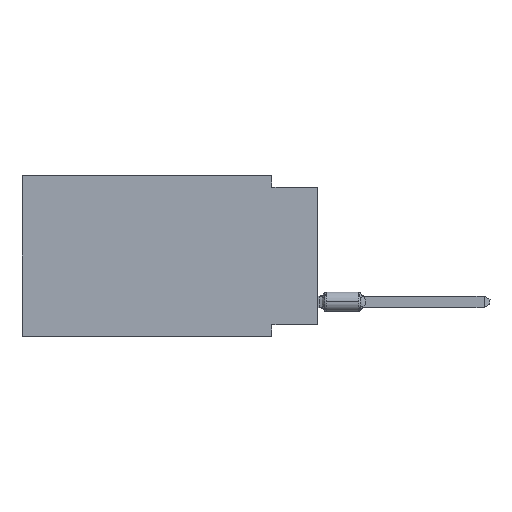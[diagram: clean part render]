
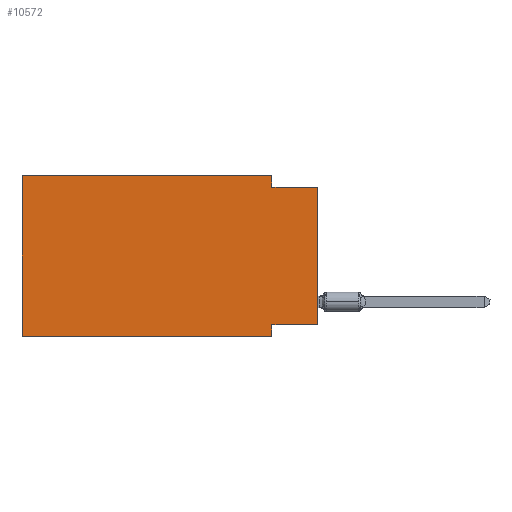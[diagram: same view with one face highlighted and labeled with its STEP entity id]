
A CAD part, left-side view. The second image highlights one B-rep face of the part: STEP entity #10572.
In plain terms, the highlighted planar face has unit normal (-1, 0, 0).
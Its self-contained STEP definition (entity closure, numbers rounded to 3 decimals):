
#329 = ORIENTED_EDGE ( 'NONE', *, *, #6114, .F. ) ;
#691 = DIRECTION ( 'NONE',  ( 1., 0., 0. ) ) ;
#1422 = CARTESIAN_POINT ( 'NONE',  ( 0., 0., -8.255 ) ) ;
#1438 = DIRECTION ( 'NONE',  ( 0., 0., 1. ) ) ;
#2077 = CARTESIAN_POINT ( 'NONE',  ( 0., 2.54, -0.635 ) ) ;
#2376 = EDGE_CURVE ( 'NONE', #9043, #14694, #4723, .T. ) ;
#2494 = VERTEX_POINT ( 'NONE', #3031 ) ;
#2720 = CARTESIAN_POINT ( 'NONE',  ( 0., 2.54, 0. ) ) ;
#2972 = LINE ( 'NONE', #18921, #23344 ) ;
#3031 = CARTESIAN_POINT ( 'NONE',  ( 0., 0., -8.255 ) ) ;
#3110 = FACE_OUTER_BOUND ( 'NONE', #8371, .T. ) ;
#3213 = VECTOR ( 'NONE', #9272, 1000. ) ;
#3931 = VECTOR ( 'NONE', #1438, 1000. ) ;
#4723 = LINE ( 'NONE', #12190, #16161 ) ;
#4898 = LINE ( 'NONE', #2720, #10779 ) ;
#5669 = DIRECTION ( 'NONE',  ( 0., 0., -1. ) ) ;
#5907 = VECTOR ( 'NONE', #14021, 1000. ) ;
#6093 = CARTESIAN_POINT ( 'NONE',  ( 0., 16.383, 0. ) ) ;
#6114 = EDGE_CURVE ( 'NONE', #9939, #9043, #4898, .T. ) ;
#6297 = LINE ( 'NONE', #21862, #5907 ) ;
#7041 = VERTEX_POINT ( 'NONE', #6093 ) ;
#7837 = ORIENTED_EDGE ( 'NONE', *, *, #2376, .F. ) ;
#8371 = EDGE_LOOP ( 'NONE', ( #8626, #7837, #329, #10147, #17397, #13687, #11802, #23444 ) ) ;
#8626 = ORIENTED_EDGE ( 'NONE', *, *, #24966, .T. ) ;
#9043 = VERTEX_POINT ( 'NONE', #2077 ) ;
#9272 = DIRECTION ( 'NONE',  ( 0., 1., 0. ) ) ;
#9939 = VERTEX_POINT ( 'NONE', #10362 ) ;
#10147 = ORIENTED_EDGE ( 'NONE', *, *, #15871, .F. ) ;
#10362 = CARTESIAN_POINT ( 'NONE',  ( 0., 2.54, 0. ) ) ;
#10436 = VECTOR ( 'NONE', #5669, 1000. ) ;
#10572 = ADVANCED_FACE ( 'NONE', ( #3110 ), #14825, .F. ) ;
#10779 = VECTOR ( 'NONE', #20582, 1000. ) ;
#11505 = CARTESIAN_POINT ( 'NONE',  ( 0., 0., 0. ) ) ;
#11729 = LINE ( 'NONE', #24979, #3931 ) ;
#11802 = ORIENTED_EDGE ( 'NONE', *, *, #15837, .F. ) ;
#12190 = CARTESIAN_POINT ( 'NONE',  ( 0., 0., -0.635 ) ) ;
#12318 = DIRECTION ( 'NONE',  ( 0., -1., 0. ) ) ;
#12362 = AXIS2_PLACEMENT_3D ( 'NONE', #18318, #691, #22916 ) ;
#13174 = CARTESIAN_POINT ( 'NONE',  ( 0., 2.54, -8.255 ) ) ;
#13687 = ORIENTED_EDGE ( 'NONE', *, *, #20154, .T. ) ;
#14021 = DIRECTION ( 'NONE',  ( 0., -1., 0. ) ) ;
#14225 = VECTOR ( 'NONE', #21532, 1000. ) ;
#14694 = VERTEX_POINT ( 'NONE', #21346 ) ;
#14825 = PLANE ( 'NONE',  #12362 ) ;
#15498 = LINE ( 'NONE', #11505, #14225 ) ;
#15837 = EDGE_CURVE ( 'NONE', #16480, #24298, #21350, .T. ) ;
#15871 = EDGE_CURVE ( 'NONE', #7041, #9939, #6297, .T. ) ;
#16161 = VECTOR ( 'NONE', #12318, 1000. ) ;
#16480 = VERTEX_POINT ( 'NONE', #13174 ) ;
#16754 = DIRECTION ( 'NONE',  ( 0., -1., 0. ) ) ;
#17397 = ORIENTED_EDGE ( 'NONE', *, *, #25268, .F. ) ;
#18318 = CARTESIAN_POINT ( 'NONE',  ( 0., 16.383, 0. ) ) ;
#18921 = CARTESIAN_POINT ( 'NONE',  ( 0., 16.383, -8.89 ) ) ;
#19044 = LINE ( 'NONE', #1422, #3213 ) ;
#20071 = CARTESIAN_POINT ( 'NONE',  ( 0., 2.54, -8.89 ) ) ;
#20154 = EDGE_CURVE ( 'NONE', #22149, #24298, #2972, .T. ) ;
#20308 = EDGE_CURVE ( 'NONE', #2494, #16480, #19044, .T. ) ;
#20582 = DIRECTION ( 'NONE',  ( 0., 0., -1. ) ) ;
#21346 = CARTESIAN_POINT ( 'NONE',  ( 0., 0., -0.635 ) ) ;
#21350 = LINE ( 'NONE', #23032, #10436 ) ;
#21532 = DIRECTION ( 'NONE',  ( 0., 0., 1. ) ) ;
#21862 = CARTESIAN_POINT ( 'NONE',  ( 0., 16.383, 0. ) ) ;
#22149 = VERTEX_POINT ( 'NONE', #22723 ) ;
#22723 = CARTESIAN_POINT ( 'NONE',  ( 0., 16.383, -8.89 ) ) ;
#22916 = DIRECTION ( 'NONE',  ( 0., 0., -1. ) ) ;
#23032 = CARTESIAN_POINT ( 'NONE',  ( 0., 2.54, -8.89 ) ) ;
#23344 = VECTOR ( 'NONE', #16754, 1000. ) ;
#23444 = ORIENTED_EDGE ( 'NONE', *, *, #20308, .F. ) ;
#24298 = VERTEX_POINT ( 'NONE', #20071 ) ;
#24966 = EDGE_CURVE ( 'NONE', #2494, #14694, #15498, .T. ) ;
#24979 = CARTESIAN_POINT ( 'NONE',  ( 0., 16.383, 0. ) ) ;
#25268 = EDGE_CURVE ( 'NONE', #22149, #7041, #11729, .T. ) ;
